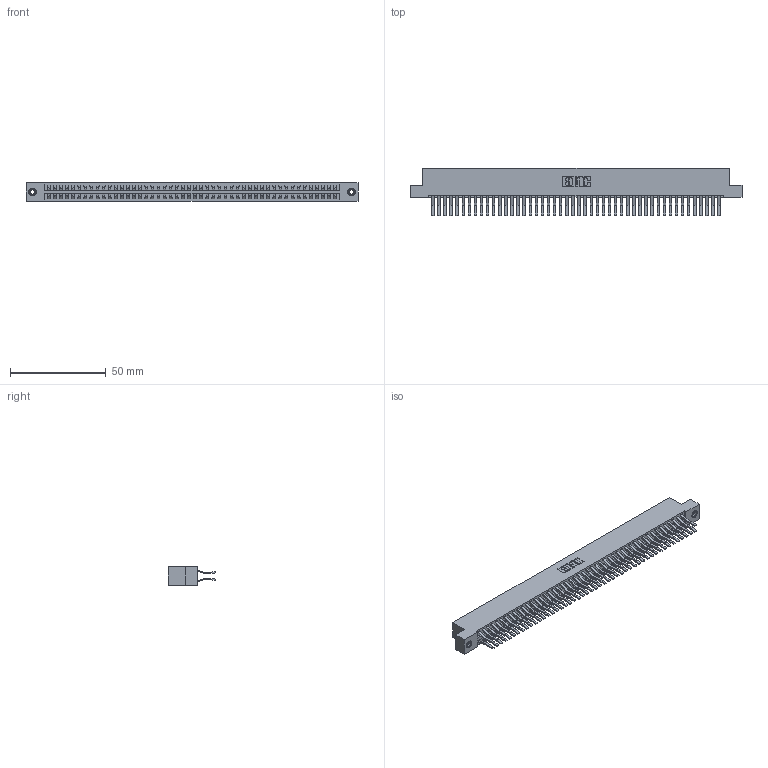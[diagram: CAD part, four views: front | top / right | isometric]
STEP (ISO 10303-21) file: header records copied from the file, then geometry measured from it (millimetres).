
FILE_DESCRIPTION (( 'STEP AP203' ), '1' );
FILE_NAME ('346-096-560-208.STEP', '2022-05-26T17:21:42', ( '' ), ( '' ), 'SwSTEP 2.0', 'SolidWorks 2020', '' );
FILE_SCHEMA (( 'CONFIG_CONTROL_DESIGN' ));
Length unit declared in the file: inch
Products named in the file (4): 346 Part_Flush Mounting Lugs - 0.156 Dia-TI; 346-096-560-208; 345-292-001_560 Tail; 345-250-001_345-250-003-102
Assembly tree (99 placements, depth 2):
  346-096-560-208
    346 Part_Flush Mounting Lugs - 0.156 Dia-TI
    345-292-001_560 Tail  x96
    345-250-001_345-250-003-102  x2
Bounding box: 172.97 x 24.78 x 9.4 mm (x, y, z)
Volume: 17536.4 mm3; surface area: 25898.1 mm2
Topology: 99 solids, 99 shells, 5366 faces, 15921 edges, 10478 vertices
Faces by surface type: plane 3468, cylinder 1882, cone 12, torus 4
Entity records: 31792 total; most frequent: CARTESIAN_POINT 5215, ORIENTED_EDGE 5142, DIRECTION 4677, EDGE_CURVE 2571, LINE 2223, VECTOR 2223, VERTEX_POINT 1708, AXIS2_PLACEMENT_3D 1227
